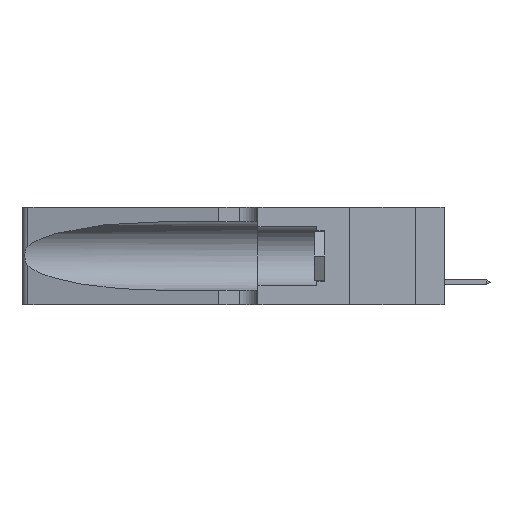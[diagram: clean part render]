
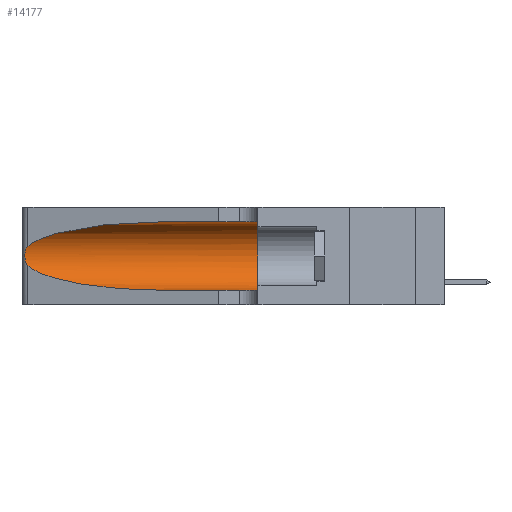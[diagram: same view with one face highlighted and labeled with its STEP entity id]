
A CAD part, left-side view. The second image highlights one B-rep face of the part: STEP entity #14177.
In plain terms, the highlighted cylindrical face has radius 3.308 mm (diameter 6.617 mm), a partial arc.
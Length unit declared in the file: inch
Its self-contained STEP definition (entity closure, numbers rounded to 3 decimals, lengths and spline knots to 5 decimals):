
#31 = DIRECTION ( 'NONE',  ( 0., -1., 0. ) ) ;
#95 = VECTOR ( 'NONE', #5670, 39.37008 ) ;
#439 = VERTEX_POINT ( 'NONE', #22974 ) ;
#1250 = CARTESIAN_POINT ( 'NONE',  ( 0.1305, 0.35, 0.31525 ) ) ;
#1501 = CARTESIAN_POINT ( 'NONE',  ( 0.1305, 1.61858, 0.31525 ) ) ;
#1957 = VERTEX_POINT ( 'NONE', #9460 ) ;
#2543 = CARTESIAN_POINT ( 'NONE',  ( 0.26075, 1.23896, 0.19203 ) ) ;
#3045 = VERTEX_POINT ( 'NONE', #6255 ) ;
#3265 = B_SPLINE_CURVE_WITH_KNOTS ( 'NONE', 3,
 ( #10230, #12600, #14531, #6464, #18469, #12251, #2543, #12335, #6558, #10312, #20604, #20344, #14453, #22609 ),
 .UNSPECIFIED., .F., .F.,
 ( 4, 2, 2, 2, 2, 2, 4 ),
 ( 0., 0.00027, 0.00053, 0.00107, 0.0016, 0.00187, 0.00214 ),
 .UNSPECIFIED. ) ;
#3641 = CARTESIAN_POINT ( 'NONE',  ( 0.1305, 0.72297, 0.05475 ) ) ;
#4089 = CARTESIAN_POINT ( 'NONE',  ( 0.25487, 1.22718, 0.14631 ) ) ;
#5078 = EDGE_CURVE ( 'NONE', #439, #16718, #23666, .T. ) ;
#5670 = DIRECTION ( 'NONE',  ( 0., -1., 0. ) ) ;
#5677 = CARTESIAN_POINT ( 'NONE',  ( 0.1305, 0.35, 0.05475 ) ) ;
#5703 = EDGE_CURVE ( 'NONE', #3045, #20987, #21115, .T. ) ;
#6255 = CARTESIAN_POINT ( 'NONE',  ( 0.1305, 0.72297, 0.31525 ) ) ;
#6464 = CARTESIAN_POINT ( 'NONE',  ( 0.25787, 1.23484, 0.2124 ) ) ;
#6558 = CARTESIAN_POINT ( 'NONE',  ( 0.26017, 1.23833, 0.17102 ) ) ;
#7510 = CARTESIAN_POINT ( 'NONE',  ( 0.25487, 1.22718, 0.14631 ) ) ;
#7816 = CARTESIAN_POINT ( 'NONE',  ( 0.2373, 1.15595, 0.08982 ) ) ;
#7833 = ORIENTED_EDGE ( 'NONE', *, *, #16251, .F. ) ;
#9460 = CARTESIAN_POINT ( 'NONE',  ( 0.25487, 1.22718, 0.22369 ) ) ;
#9668 = CARTESIAN_POINT ( 'NONE',  ( 0.18966, 0.96281, 0.05475 ) ) ;
#9796 = ORIENTED_EDGE ( 'NONE', *, *, #5703, .F. ) ;
#9979 = CARTESIAN_POINT ( 'NONE',  ( 0.1305, 1.61858, 0.05475 ) ) ;
#10230 = CARTESIAN_POINT ( 'NONE',  ( 0.25487, 1.22718, 0.22369 ) ) ;
#10312 = CARTESIAN_POINT ( 'NONE',  ( 0.25856, 1.23593, 0.16098 ) ) ;
#10984 = DIRECTION ( 'NONE',  ( 0., 1., 0. ) ) ;
#12251 = CARTESIAN_POINT ( 'NONE',  ( 0.26018, 1.23835, 0.19895 ) ) ;
#12335 = CARTESIAN_POINT ( 'NONE',  ( 0.26075, 1.23896, 0.178 ) ) ;
#12600 = CARTESIAN_POINT ( 'NONE',  ( 0.25555, 1.22994, 0.2215 ) ) ;
#12610 = CARTESIAN_POINT ( 'NONE',  ( 0.2373, 1.15595, 0.28018 ) ) ;
#13065 = EDGE_CURVE ( 'NONE', #1957, #23257, #3265, .T. ) ;
#13718 = EDGE_CURVE ( 'NONE', #3045, #1957, #24645, .T. ) ;
#14177 = ADVANCED_FACE ( 'NONE', ( #21240 ), #25650, .F. ) ;
#14397 = DIRECTION ( 'NONE',  ( 0., -1., 0. ) ) ;
#14453 = CARTESIAN_POINT ( 'NONE',  ( 0.25555, 1.22993, 0.14849 ) ) ;
#14531 = CARTESIAN_POINT ( 'NONE',  ( 0.25639, 1.23184, 0.21858 ) ) ;
#16251 = EDGE_CURVE ( 'NONE', #20987, #16718, #22453, .T. ) ;
#16517 = ORIENTED_EDGE ( 'NONE', *, *, #5078, .T. ) ;
#16718 = VERTEX_POINT ( 'NONE', #5677 ) ;
#16834 = CARTESIAN_POINT ( 'NONE',  ( 0.25487, 1.22718, 0.22369 ) ) ;
#17516 = ORIENTED_EDGE ( 'NONE', *, *, #19345, .T. ) ;
#18469 = CARTESIAN_POINT ( 'NONE',  ( 0.25854, 1.2359, 0.20912 ) ) ;
#19226 = CARTESIAN_POINT ( 'NONE',  ( 0.1305, 0.35, 0.185 ) ) ;
#19345 = EDGE_CURVE ( 'NONE', #23257, #439, #25805, .T. ) ;
#19571 = EDGE_LOOP ( 'NONE', ( #25320, #22047, #17516, #16517, #7833, #9796 ) ) ;
#20344 = CARTESIAN_POINT ( 'NONE',  ( 0.25639, 1.23186, 0.15144 ) ) ;
#20604 = CARTESIAN_POINT ( 'NONE',  ( 0.25789, 1.23486, 0.15765 ) ) ;
#20987 = VERTEX_POINT ( 'NONE', #1250 ) ;
#21115 = LINE ( 'NONE', #1501, #95 ) ;
#21240 = FACE_OUTER_BOUND ( 'NONE', #19571, .T. ) ;
#22047 = ORIENTED_EDGE ( 'NONE', *, *, #13065, .T. ) ;
#22083 = VECTOR ( 'NONE', #31, 39.37008 ) ;
#22315 = AXIS2_PLACEMENT_3D ( 'NONE', #22382, #14397, #24495 ) ;
#22382 = CARTESIAN_POINT ( 'NONE',  ( 0.1305, 1.61858, 0.185 ) ) ;
#22453 = CIRCLE ( 'NONE', #24202, 0.13025 ) ;
#22609 = CARTESIAN_POINT ( 'NONE',  ( 0.25487, 1.22718, 0.14631 ) ) ;
#22891 = CARTESIAN_POINT ( 'NONE',  ( 0.18966, 0.96281, 0.31525 ) ) ;
#22974 = CARTESIAN_POINT ( 'NONE',  ( 0.1305, 0.72297, 0.05475 ) ) ;
#23257 = VERTEX_POINT ( 'NONE', #4089 ) ;
#23666 = LINE ( 'NONE', #9979, #22083 ) ;
#24202 = AXIS2_PLACEMENT_3D ( 'NONE', #19226, #10984, #25047 ) ;
#24495 = DIRECTION ( 'NONE',  ( 0., 0., -1. ) ) ;
#24645 =( BOUNDED_CURVE ( )  B_SPLINE_CURVE ( 3, ( #24745, #22891, #12610, #16834 ),
 .UNSPECIFIED., .F., .F. ) 
 B_SPLINE_CURVE_WITH_KNOTS ( ( 4, 4 ),
 ( 1.5708, 2.84003 ),
 .UNSPECIFIED. ) 
 CURVE ( )  GEOMETRIC_REPRESENTATION_ITEM ( )  RATIONAL_B_SPLINE_CURVE ( ( 1., 0.87, 0.87, 1. ) ) 
 REPRESENTATION_ITEM ( '' )  );
#24745 = CARTESIAN_POINT ( 'NONE',  ( 0.1305, 0.72297, 0.31525 ) ) ;
#25047 = DIRECTION ( 'NONE',  ( 0., 0., 1. ) ) ;
#25320 = ORIENTED_EDGE ( 'NONE', *, *, #13718, .T. ) ;
#25650 = CYLINDRICAL_SURFACE ( 'NONE', #22315, 0.13025 ) ;
#25805 =( BOUNDED_CURVE ( )  B_SPLINE_CURVE ( 3, ( #7510, #7816, #9668, #3641 ),
 .UNSPECIFIED., .F., .F. ) 
 B_SPLINE_CURVE_WITH_KNOTS ( ( 4, 4 ),
 ( 3.44316, 4.71239 ),
 .UNSPECIFIED. ) 
 CURVE ( )  GEOMETRIC_REPRESENTATION_ITEM ( )  RATIONAL_B_SPLINE_CURVE ( ( 1., 0.87, 0.87, 1. ) ) 
 REPRESENTATION_ITEM ( '' )  );
